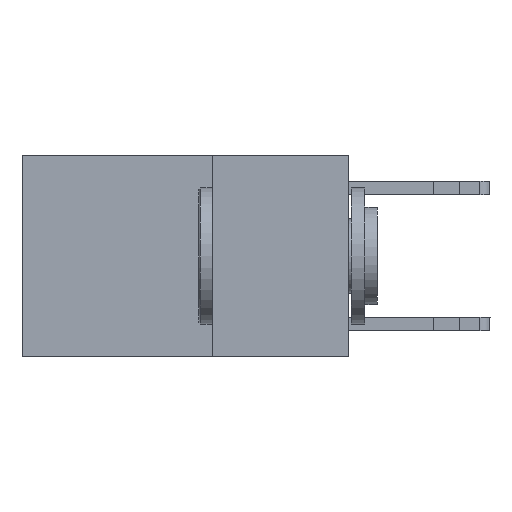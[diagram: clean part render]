
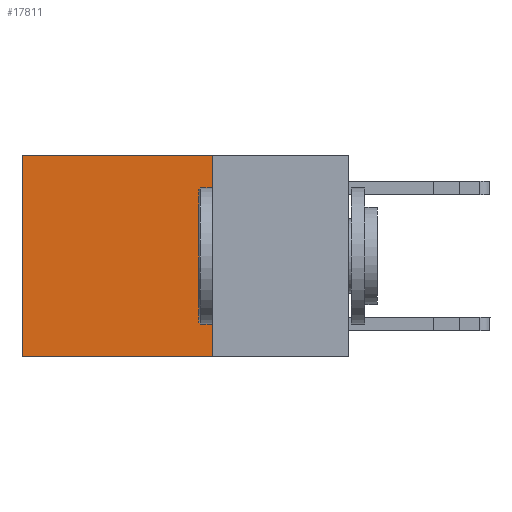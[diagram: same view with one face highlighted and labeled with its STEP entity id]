
A CAD part, left-side view. The second image highlights one B-rep face of the part: STEP entity #17811.
In plain terms, the highlighted planar face has unit normal (-1, 0, 0).
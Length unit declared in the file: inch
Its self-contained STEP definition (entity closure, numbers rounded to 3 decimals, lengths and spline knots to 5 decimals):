
#1197 = DIRECTION ( 'NONE',  ( 0., 0., -1. ) ) ;
#2244 = CARTESIAN_POINT ( 'NONE',  ( 0.2625, 0.25, -0.37 ) ) ;
#4366 = EDGE_CURVE ( 'NONE', #17164, #18559, #9208, .T. ) ;
#4453 = DIRECTION ( 'NONE',  ( 0., 1., 0. ) ) ;
#4509 = CARTESIAN_POINT ( 'NONE',  ( 0.2625, 0.25, 0. ) ) ;
#5131 = CARTESIAN_POINT ( 'NONE',  ( 0.2625, 0.6, 0. ) ) ;
#5384 = VERTEX_POINT ( 'NONE', #10308 ) ;
#6104 = EDGE_CURVE ( 'NONE', #18559, #5384, #13692, .T. ) ;
#6304 = LINE ( 'NONE', #4509, #6485 ) ;
#6390 = ORIENTED_EDGE ( 'NONE', *, *, #22086, .T. ) ;
#6485 = VECTOR ( 'NONE', #4453, 39.37008 ) ;
#7375 = EDGE_LOOP ( 'NONE', ( #6390, #19846, #9261, #16584 ) ) ;
#9044 = VECTOR ( 'NONE', #21399, 39.37008 ) ;
#9208 = LINE ( 'NONE', #21262, #9044 ) ;
#9261 = ORIENTED_EDGE ( 'NONE', *, *, #4366, .F. ) ;
#9717 = CARTESIAN_POINT ( 'NONE',  ( 0.2625, 0.25, 0. ) ) ;
#10308 = CARTESIAN_POINT ( 'NONE',  ( 0.2625, 0.6, -0.37 ) ) ;
#13692 = LINE ( 'NONE', #18546, #14381 ) ;
#14381 = VECTOR ( 'NONE', #18486, 39.37008 ) ;
#14727 = AXIS2_PLACEMENT_3D ( 'NONE', #16378, #15779, #15724 ) ;
#15175 = VECTOR ( 'NONE', #1197, 39.37008 ) ;
#15238 = LINE ( 'NONE', #5131, #15175 ) ;
#15256 = CARTESIAN_POINT ( 'NONE',  ( 0.2625, 0.6, 0. ) ) ;
#15724 = DIRECTION ( 'NONE',  ( 0., 0., -1. ) ) ;
#15779 = DIRECTION ( 'NONE',  ( 1., 0., 0. ) ) ;
#16014 = PLANE ( 'NONE',  #14727 ) ;
#16378 = CARTESIAN_POINT ( 'NONE',  ( 0.2625, 0.25, 0. ) ) ;
#16584 = ORIENTED_EDGE ( 'NONE', *, *, #19785, .T. ) ;
#17164 = VERTEX_POINT ( 'NONE', #9717 ) ;
#17811 = ADVANCED_FACE ( 'NONE', ( #20748 ), #16014, .F. ) ;
#18486 = DIRECTION ( 'NONE',  ( 0., 1., 0. ) ) ;
#18546 = CARTESIAN_POINT ( 'NONE',  ( 0.2625, 0.25, -0.37 ) ) ;
#18559 = VERTEX_POINT ( 'NONE', #2244 ) ;
#19785 = EDGE_CURVE ( 'NONE', #17164, #20768, #6304, .T. ) ;
#19846 = ORIENTED_EDGE ( 'NONE', *, *, #6104, .F. ) ;
#20748 = FACE_OUTER_BOUND ( 'NONE', #7375, .T. ) ;
#20768 = VERTEX_POINT ( 'NONE', #15256 ) ;
#21262 = CARTESIAN_POINT ( 'NONE',  ( 0.2625, 0.25, 0. ) ) ;
#21399 = DIRECTION ( 'NONE',  ( 0., 0., -1. ) ) ;
#22086 = EDGE_CURVE ( 'NONE', #20768, #5384, #15238, .T. ) ;
